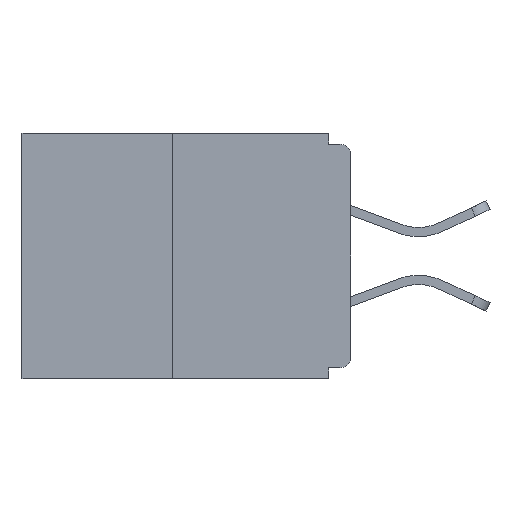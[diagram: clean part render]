
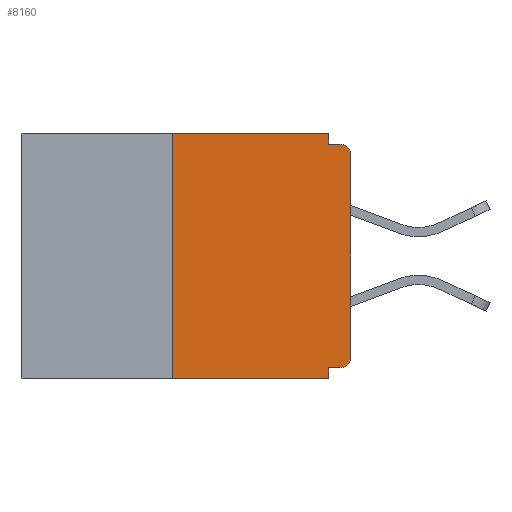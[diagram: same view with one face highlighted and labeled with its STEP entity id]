
A CAD part, left-side view. The second image highlights one B-rep face of the part: STEP entity #8160.
In plain terms, the highlighted planar face has unit normal (-1, 0, 0).
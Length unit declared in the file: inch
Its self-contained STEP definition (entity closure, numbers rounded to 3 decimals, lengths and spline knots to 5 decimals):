
#509 = CARTESIAN_POINT ( 'NONE',  ( 0., 0., -0.03 ) ) ;
#619 = LINE ( 'NONE', #9026, #9410 ) ;
#754 = DIRECTION ( 'NONE',  ( 0., 0., 1. ) ) ;
#985 = DIRECTION ( 'NONE',  ( 0., 0., -1. ) ) ;
#1227 = DIRECTION ( 'NONE',  ( 0., 0., -1. ) ) ;
#1275 = CIRCLE ( 'NONE', #6810, 0.015 ) ;
#1302 = EDGE_CURVE ( 'NONE', #7334, #6235, #2030, .T. ) ;
#1413 = DIRECTION ( 'NONE',  ( 0., 0., -1. ) ) ;
#1597 = DIRECTION ( 'NONE',  ( 0., -1., 0. ) ) ;
#1629 = ORIENTED_EDGE ( 'NONE', *, *, #1302, .F. ) ;
#1921 = EDGE_CURVE ( 'NONE', #4514, #11551, #1275, .T. ) ;
#2030 = LINE ( 'NONE', #4499, #3049 ) ;
#2225 = VERTEX_POINT ( 'NONE', #8465 ) ;
#2545 = CARTESIAN_POINT ( 'NONE',  ( 0., 0.015, -0.03 ) ) ;
#2614 = ORIENTED_EDGE ( 'NONE', *, *, #7125, .T. ) ;
#2619 = ORIENTED_EDGE ( 'NONE', *, *, #11969, .F. ) ;
#3049 = VECTOR ( 'NONE', #6450, 39.37008 ) ;
#3379 = CARTESIAN_POINT ( 'NONE',  ( 0., 0., -0.015 ) ) ;
#3758 = EDGE_CURVE ( 'NONE', #6235, #9693, #5526, .T. ) ;
#4098 = DIRECTION ( 'NONE',  ( 0., -1., 0. ) ) ;
#4273 = CARTESIAN_POINT ( 'NONE',  ( 0., 0.031, 0. ) ) ;
#4386 = CARTESIAN_POINT ( 'NONE',  ( 0., 0., -0.328 ) ) ;
#4410 = EDGE_CURVE ( 'NONE', #7334, #11316, #7428, .T. ) ;
#4415 = EDGE_CURVE ( 'NONE', #2225, #11551, #7589, .T. ) ;
#4499 = CARTESIAN_POINT ( 'NONE',  ( 0., 0.25, 0. ) ) ;
#4514 = VERTEX_POINT ( 'NONE', #509 ) ;
#4520 = DIRECTION ( 'NONE',  ( 0., 0., -1. ) ) ;
#4649 = LINE ( 'NONE', #4386, #12222 ) ;
#4724 = DIRECTION ( 'NONE',  ( 1., 0., 0. ) ) ;
#4920 = EDGE_CURVE ( 'NONE', #7057, #11316, #8035, .T. ) ;
#4937 = VECTOR ( 'NONE', #4098, 39.37008 ) ;
#5110 = CARTESIAN_POINT ( 'NONE',  ( 0., 0., -0.313 ) ) ;
#5211 = ORIENTED_EDGE ( 'NONE', *, *, #1921, .T. ) ;
#5334 = CARTESIAN_POINT ( 'NONE',  ( 0., 0.031, -0.328 ) ) ;
#5339 = DIRECTION ( 'NONE',  ( 0., -1., 0. ) ) ;
#5526 = LINE ( 'NONE', #7902, #4937 ) ;
#5757 = EDGE_CURVE ( 'NONE', #7251, #10240, #11036, .T. ) ;
#5876 = ORIENTED_EDGE ( 'NONE', *, *, #3758, .F. ) ;
#6132 = ORIENTED_EDGE ( 'NONE', *, *, #10726, .F. ) ;
#6183 = ORIENTED_EDGE ( 'NONE', *, *, #4920, .F. ) ;
#6235 = VERTEX_POINT ( 'NONE', #12244 ) ;
#6321 = AXIS2_PLACEMENT_3D ( 'NONE', #10446, #4724, #985 ) ;
#6355 = DIRECTION ( 'NONE',  ( -1., 0., 0. ) ) ;
#6450 = DIRECTION ( 'NONE',  ( 0., 0., 1. ) ) ;
#6730 = EDGE_LOOP ( 'NONE', ( #5876, #1629, #7557, #6183, #6132, #9631, #2614, #5211, #7978, #2619 ) ) ;
#6810 = AXIS2_PLACEMENT_3D ( 'NONE', #2545, #6355, #4520 ) ;
#7057 = VERTEX_POINT ( 'NONE', #5334 ) ;
#7125 = EDGE_CURVE ( 'NONE', #10240, #4514, #9493, .T. ) ;
#7251 = VERTEX_POINT ( 'NONE', #7611 ) ;
#7334 = VERTEX_POINT ( 'NONE', #11703 ) ;
#7428 = LINE ( 'NONE', #8019, #12194 ) ;
#7557 = ORIENTED_EDGE ( 'NONE', *, *, #4410, .T. ) ;
#7589 = LINE ( 'NONE', #3379, #9684 ) ;
#7611 = CARTESIAN_POINT ( 'NONE',  ( 0., 0.015, -0.328 ) ) ;
#7902 = CARTESIAN_POINT ( 'NONE',  ( 0., 0.46, 0. ) ) ;
#7978 = ORIENTED_EDGE ( 'NONE', *, *, #4415, .F. ) ;
#8019 = CARTESIAN_POINT ( 'NONE',  ( 0., 0.46, -0.343 ) ) ;
#8035 = LINE ( 'NONE', #11711, #11317 ) ;
#8160 = ADVANCED_FACE ( 'NONE', ( #10066 ), #12231, .F. ) ;
#8465 = CARTESIAN_POINT ( 'NONE',  ( 0., 0.031, -0.015 ) ) ;
#8706 = DIRECTION ( 'NONE',  ( -1., 0., 0. ) ) ;
#8899 = VECTOR ( 'NONE', #754, 39.37008 ) ;
#9026 = CARTESIAN_POINT ( 'NONE',  ( 0., 0.031, 0. ) ) ;
#9410 = VECTOR ( 'NONE', #1413, 39.37008 ) ;
#9493 = LINE ( 'NONE', #11250, #8899 ) ;
#9498 = DIRECTION ( 'NONE',  ( 0., 0., -1. ) ) ;
#9569 = AXIS2_PLACEMENT_3D ( 'NONE', #10633, #8706, #9498 ) ;
#9631 = ORIENTED_EDGE ( 'NONE', *, *, #5757, .T. ) ;
#9684 = VECTOR ( 'NONE', #5339, 39.37008 ) ;
#9693 = VERTEX_POINT ( 'NONE', #4273 ) ;
#10066 = FACE_OUTER_BOUND ( 'NONE', #6730, .T. ) ;
#10240 = VERTEX_POINT ( 'NONE', #5110 ) ;
#10408 = CARTESIAN_POINT ( 'NONE',  ( 0., 0.015, -0.015 ) ) ;
#10446 = CARTESIAN_POINT ( 'NONE',  ( 0., 0.46, 0. ) ) ;
#10633 = CARTESIAN_POINT ( 'NONE',  ( 0., 0.015, -0.313 ) ) ;
#10726 = EDGE_CURVE ( 'NONE', #7251, #7057, #4649, .T. ) ;
#11036 = CIRCLE ( 'NONE', #9569, 0.015 ) ;
#11075 = CARTESIAN_POINT ( 'NONE',  ( 0., 0.031, -0.343 ) ) ;
#11109 = DIRECTION ( 'NONE',  ( 0., 1., 0. ) ) ;
#11250 = CARTESIAN_POINT ( 'NONE',  ( 0., 0., 0. ) ) ;
#11316 = VERTEX_POINT ( 'NONE', #11075 ) ;
#11317 = VECTOR ( 'NONE', #1227, 39.37008 ) ;
#11551 = VERTEX_POINT ( 'NONE', #10408 ) ;
#11703 = CARTESIAN_POINT ( 'NONE',  ( 0., 0.25, -0.343 ) ) ;
#11711 = CARTESIAN_POINT ( 'NONE',  ( 0., 0.031, -0.343 ) ) ;
#11969 = EDGE_CURVE ( 'NONE', #9693, #2225, #619, .T. ) ;
#12194 = VECTOR ( 'NONE', #1597, 39.37008 ) ;
#12222 = VECTOR ( 'NONE', #11109, 39.37008 ) ;
#12231 = PLANE ( 'NONE',  #6321 ) ;
#12244 = CARTESIAN_POINT ( 'NONE',  ( 0., 0.25, 0. ) ) ;
